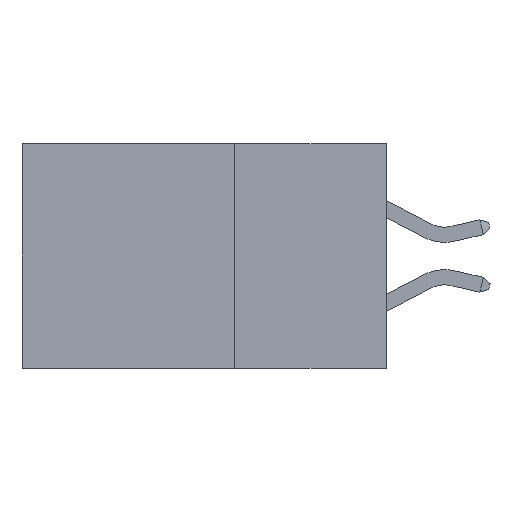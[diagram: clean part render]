
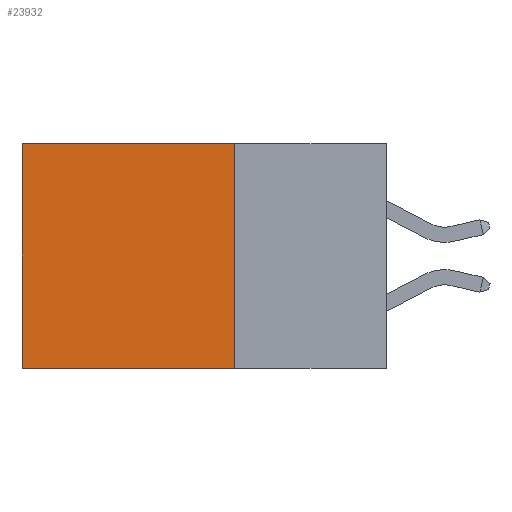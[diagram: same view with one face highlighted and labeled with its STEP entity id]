
A CAD part, left-side view. The second image highlights one B-rep face of the part: STEP entity #23932.
In plain terms, the highlighted planar face has unit normal (-1, 0, 0).
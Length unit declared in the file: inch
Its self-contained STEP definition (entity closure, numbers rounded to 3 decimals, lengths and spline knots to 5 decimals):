
#34 = CARTESIAN_POINT ( 'NONE',  ( 0.298, 0.6, 0. ) ) ;
#863 = EDGE_LOOP ( 'NONE', ( #5290, #6805, #7808, #24194 ) ) ;
#1533 = DIRECTION ( 'NONE',  ( 0., 1., 0. ) ) ;
#1813 = CARTESIAN_POINT ( 'NONE',  ( 0.298, 0.25, -0.37 ) ) ;
#1824 = CARTESIAN_POINT ( 'NONE',  ( 0.298, 0.6, 0. ) ) ;
#1870 = VECTOR ( 'NONE', #18070, 39.37008 ) ;
#2131 = VECTOR ( 'NONE', #2394, 39.37008 ) ;
#2247 = DIRECTION ( 'NONE',  ( 0., 0., -1. ) ) ;
#2394 = DIRECTION ( 'NONE',  ( 0., 1., 0. ) ) ;
#3800 = LINE ( 'NONE', #34, #11762 ) ;
#5051 = VECTOR ( 'NONE', #1533, 39.37008 ) ;
#5290 = ORIENTED_EDGE ( 'NONE', *, *, #13149, .T. ) ;
#6530 = PLANE ( 'NONE',  #20253 ) ;
#6805 = ORIENTED_EDGE ( 'NONE', *, *, #22855, .F. ) ;
#6859 = LINE ( 'NONE', #12715, #1870 ) ;
#7160 = LINE ( 'NONE', #19509, #2131 ) ;
#7808 = ORIENTED_EDGE ( 'NONE', *, *, #16383, .F. ) ;
#8275 = VERTEX_POINT ( 'NONE', #1813 ) ;
#8306 = CARTESIAN_POINT ( 'NONE',  ( 0.298, 0.25, 0. ) ) ;
#8313 = CARTESIAN_POINT ( 'NONE',  ( 0.298, 0.6, -0.37 ) ) ;
#10360 = DIRECTION ( 'NONE',  ( 0., 0., -1. ) ) ;
#10442 = CARTESIAN_POINT ( 'NONE',  ( 0.298, 0.25, 0. ) ) ;
#11699 = FACE_OUTER_BOUND ( 'NONE', #863, .T. ) ;
#11762 = VECTOR ( 'NONE', #2247, 39.37008 ) ;
#12715 = CARTESIAN_POINT ( 'NONE',  ( 0.298, 0.25, 0. ) ) ;
#13149 = EDGE_CURVE ( 'NONE', #19260, #17552, #3800, .T. ) ;
#13279 = LINE ( 'NONE', #23441, #5051 ) ;
#14263 = DIRECTION ( 'NONE',  ( 1., 0., 0. ) ) ;
#16383 = EDGE_CURVE ( 'NONE', #23801, #8275, #6859, .T. ) ;
#17552 = VERTEX_POINT ( 'NONE', #8313 ) ;
#18070 = DIRECTION ( 'NONE',  ( 0., 0., -1. ) ) ;
#19260 = VERTEX_POINT ( 'NONE', #1824 ) ;
#19509 = CARTESIAN_POINT ( 'NONE',  ( 0.298, 0.25, 0. ) ) ;
#20253 = AXIS2_PLACEMENT_3D ( 'NONE', #10442, #14263, #10360 ) ;
#22084 = EDGE_CURVE ( 'NONE', #23801, #19260, #7160, .T. ) ;
#22855 = EDGE_CURVE ( 'NONE', #8275, #17552, #13279, .T. ) ;
#23441 = CARTESIAN_POINT ( 'NONE',  ( 0.298, 0.25, -0.37 ) ) ;
#23801 = VERTEX_POINT ( 'NONE', #8306 ) ;
#23932 = ADVANCED_FACE ( 'NONE', ( #11699 ), #6530, .F. ) ;
#24194 = ORIENTED_EDGE ( 'NONE', *, *, #22084, .T. ) ;
